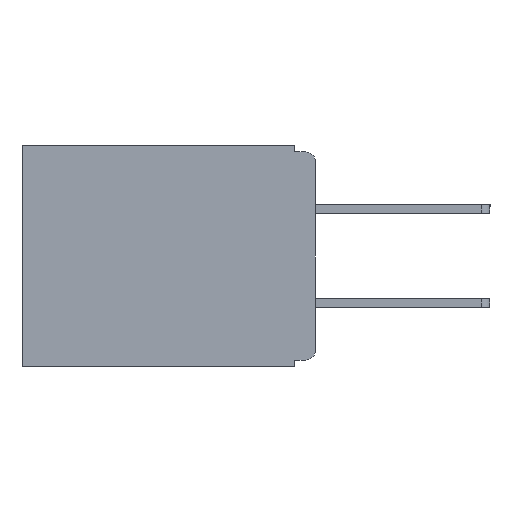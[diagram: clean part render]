
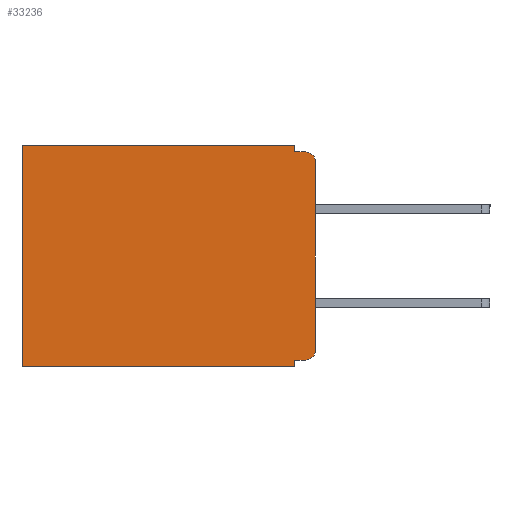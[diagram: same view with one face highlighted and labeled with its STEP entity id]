
A CAD part, left-side view. The second image highlights one B-rep face of the part: STEP entity #33236.
In plain terms, the highlighted planar face has unit normal (-1, 0, 0).
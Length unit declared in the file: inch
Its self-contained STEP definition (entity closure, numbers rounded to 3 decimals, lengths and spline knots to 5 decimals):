
#331 = VECTOR ( 'NONE', #20810, 39.37008 ) ;
#362 = CARTESIAN_POINT ( 'NONE',  ( 0.3, 0., -0.33 ) ) ;
#471 = CARTESIAN_POINT ( 'NONE',  ( 0.3, 0., 0. ) ) ;
#1193 = LINE ( 'NONE', #3512, #7174 ) ;
#1406 = ORIENTED_EDGE ( 'NONE', *, *, #9977, .F. ) ;
#1563 = CARTESIAN_POINT ( 'NONE',  ( 0.3, 0., -0.33 ) ) ;
#1667 = DIRECTION ( 'NONE',  ( 0., 1., 0. ) ) ;
#1778 = ORIENTED_EDGE ( 'NONE', *, *, #18296, .F. ) ;
#1902 = LINE ( 'NONE', #12174, #14736 ) ;
#2939 = DIRECTION ( 'NONE',  ( 0., 0., -1. ) ) ;
#3040 = DIRECTION ( 'NONE',  ( 0., 1., 0. ) ) ;
#3512 = CARTESIAN_POINT ( 'NONE',  ( 0.3, 0., -0.32 ) ) ;
#4053 = CARTESIAN_POINT ( 'NONE',  ( 0.3, 0.015, -0.305 ) ) ;
#4356 = EDGE_CURVE ( 'NONE', #20988, #13673, #24292, .T. ) ;
#4524 = ORIENTED_EDGE ( 'NONE', *, *, #15754, .F. ) ;
#4949 = VECTOR ( 'NONE', #3040, 39.37008 ) ;
#6444 = VECTOR ( 'NONE', #15674, 39.37008 ) ;
#6613 = DIRECTION ( 'NONE',  ( 0., 0., -1. ) ) ;
#7134 = LINE ( 'NONE', #18201, #331 ) ;
#7174 = VECTOR ( 'NONE', #8670, 39.37008 ) ;
#7207 = VECTOR ( 'NONE', #1667, 39.37008 ) ;
#7342 = CARTESIAN_POINT ( 'NONE',  ( 0.3, 0.031, -0.32 ) ) ;
#7354 = ORIENTED_EDGE ( 'NONE', *, *, #17643, .F. ) ;
#8184 = VECTOR ( 'NONE', #8593, 39.37008 ) ;
#8225 = VERTEX_POINT ( 'NONE', #7342 ) ;
#8425 = CARTESIAN_POINT ( 'NONE',  ( 0.3, 0.437, 0. ) ) ;
#8461 = ORIENTED_EDGE ( 'NONE', *, *, #18146, .F. ) ;
#8471 = CARTESIAN_POINT ( 'NONE',  ( 0.3, 0.015, -0.025 ) ) ;
#8593 = DIRECTION ( 'NONE',  ( 0., 0., -1. ) ) ;
#8670 = DIRECTION ( 'NONE',  ( 0., 1., 0. ) ) ;
#9105 = CARTESIAN_POINT ( 'NONE',  ( 0.3, 0.031, -0.01 ) ) ;
#9362 = VERTEX_POINT ( 'NONE', #14452 ) ;
#9671 = EDGE_CURVE ( 'NONE', #8225, #10873, #15006, .T. ) ;
#9977 = EDGE_CURVE ( 'NONE', #20988, #15726, #1902, .T. ) ;
#10669 = CARTESIAN_POINT ( 'NONE',  ( 0.3, 0.437, -0.33 ) ) ;
#10873 = VERTEX_POINT ( 'NONE', #33219 ) ;
#11549 = DIRECTION ( 'NONE',  ( 0., 0., -1. ) ) ;
#12005 = CARTESIAN_POINT ( 'NONE',  ( 0.3, 0.015, -0.01 ) ) ;
#12174 = CARTESIAN_POINT ( 'NONE',  ( 0.3, 0., -0.33 ) ) ;
#12459 = LINE ( 'NONE', #10669, #6444 ) ;
#12994 = VERTEX_POINT ( 'NONE', #8425 ) ;
#13673 = VERTEX_POINT ( 'NONE', #12005 ) ;
#14013 = EDGE_CURVE ( 'NONE', #12994, #25137, #12459, .T. ) ;
#14037 = LINE ( 'NONE', #1563, #7207 ) ;
#14400 = DIRECTION ( 'NONE',  ( 0., 0., -1. ) ) ;
#14452 = CARTESIAN_POINT ( 'NONE',  ( 0.3, 0.015, -0.32 ) ) ;
#14736 = VECTOR ( 'NONE', #25046, 39.37008 ) ;
#14847 = AXIS2_PLACEMENT_3D ( 'NONE', #362, #18331, #2939 ) ;
#15006 = LINE ( 'NONE', #21454, #8184 ) ;
#15674 = DIRECTION ( 'NONE',  ( 0., 0., -1. ) ) ;
#15700 = PLANE ( 'NONE',  #14847 ) ;
#15719 = AXIS2_PLACEMENT_3D ( 'NONE', #8471, #22095, #11549 ) ;
#15726 = VERTEX_POINT ( 'NONE', #18085 ) ;
#15754 = EDGE_CURVE ( 'NONE', #24200, #13673, #7134, .T. ) ;
#16307 = ORIENTED_EDGE ( 'NONE', *, *, #33274, .T. ) ;
#17011 = ORIENTED_EDGE ( 'NONE', *, *, #4356, .T. ) ;
#17443 = CARTESIAN_POINT ( 'NONE',  ( 0.3, 0., -0.025 ) ) ;
#17643 = EDGE_CURVE ( 'NONE', #10873, #25137, #14037, .T. ) ;
#18085 = CARTESIAN_POINT ( 'NONE',  ( 0.3, 0., -0.305 ) ) ;
#18146 = EDGE_CURVE ( 'NONE', #9362, #8225, #1193, .T. ) ;
#18201 = CARTESIAN_POINT ( 'NONE',  ( 0.3, 0., -0.01 ) ) ;
#18296 = EDGE_CURVE ( 'NONE', #30294, #24200, #22860, .T. ) ;
#18331 = DIRECTION ( 'NONE',  ( 1., 0., 0. ) ) ;
#18803 = EDGE_CURVE ( 'NONE', #9362, #15726, #22051, .T. ) ;
#19903 = AXIS2_PLACEMENT_3D ( 'NONE', #4053, #22053, #6613 ) ;
#20810 = DIRECTION ( 'NONE',  ( 0., -1., 0. ) ) ;
#20988 = VERTEX_POINT ( 'NONE', #17443 ) ;
#21441 = CARTESIAN_POINT ( 'NONE',  ( 0.3, 0.437, -0.33 ) ) ;
#21454 = CARTESIAN_POINT ( 'NONE',  ( 0.3, 0.031, -0.33 ) ) ;
#22051 = CIRCLE ( 'NONE', #19903, 0.015 ) ;
#22053 = DIRECTION ( 'NONE',  ( -1., 0., 0. ) ) ;
#22079 = VECTOR ( 'NONE', #14400, 39.37008 ) ;
#22095 = DIRECTION ( 'NONE',  ( -1., 0., 0. ) ) ;
#22512 = EDGE_LOOP ( 'NONE', ( #1406, #17011, #4524, #1778, #16307, #29418, #7354, #27234, #8461, #28680 ) ) ;
#22860 = LINE ( 'NONE', #27262, #22079 ) ;
#24200 = VERTEX_POINT ( 'NONE', #9105 ) ;
#24292 = CIRCLE ( 'NONE', #15719, 0.015 ) ;
#25046 = DIRECTION ( 'NONE',  ( 0., 0., -1. ) ) ;
#25137 = VERTEX_POINT ( 'NONE', #21441 ) ;
#25512 = FACE_OUTER_BOUND ( 'NONE', #22512, .T. ) ;
#27000 = CARTESIAN_POINT ( 'NONE',  ( 0.3, 0.031, 0. ) ) ;
#27234 = ORIENTED_EDGE ( 'NONE', *, *, #9671, .F. ) ;
#27262 = CARTESIAN_POINT ( 'NONE',  ( 0.3, 0.031, 0. ) ) ;
#28680 = ORIENTED_EDGE ( 'NONE', *, *, #18803, .T. ) ;
#29418 = ORIENTED_EDGE ( 'NONE', *, *, #14013, .T. ) ;
#30294 = VERTEX_POINT ( 'NONE', #27000 ) ;
#32340 = LINE ( 'NONE', #471, #4949 ) ;
#33219 = CARTESIAN_POINT ( 'NONE',  ( 0.3, 0.031, -0.33 ) ) ;
#33236 = ADVANCED_FACE ( 'NONE', ( #25512 ), #15700, .F. ) ;
#33274 = EDGE_CURVE ( 'NONE', #30294, #12994, #32340, .T. ) ;
